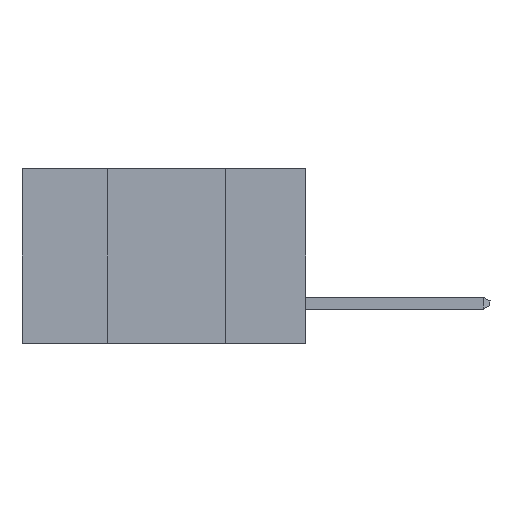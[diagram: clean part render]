
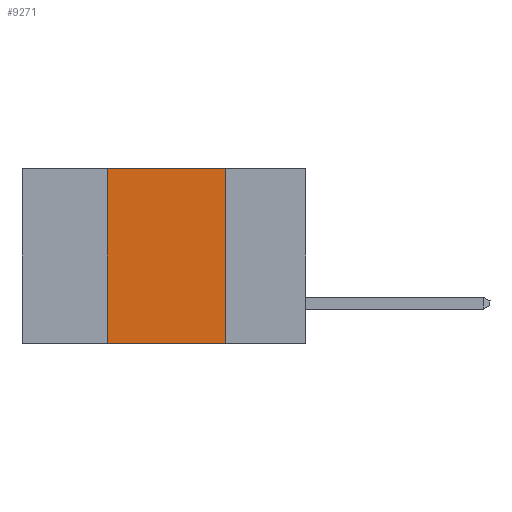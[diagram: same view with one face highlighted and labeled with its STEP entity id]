
A CAD part, left-side view. The second image highlights one B-rep face of the part: STEP entity #9271.
In plain terms, the highlighted planar face has unit normal (-1, 0, 0).
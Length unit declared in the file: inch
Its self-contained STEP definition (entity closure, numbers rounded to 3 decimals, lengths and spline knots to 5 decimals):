
#103 = DIRECTION ( 'NONE',  ( 0., 0., -1. ) ) ;
#150 = DIRECTION ( 'NONE',  ( 0., -1., 0. ) ) ;
#769 = CARTESIAN_POINT ( 'NONE',  ( 0., 0.17, -0.37 ) ) ;
#1014 = LINE ( 'NONE', #6149, #9701 ) ;
#1669 = VERTEX_POINT ( 'NONE', #7703 ) ;
#1776 = ORIENTED_EDGE ( 'NONE', *, *, #10661, .F. ) ;
#2190 = DIRECTION ( 'NONE',  ( 0., 0., 1. ) ) ;
#2389 = ORIENTED_EDGE ( 'NONE', *, *, #3791, .T. ) ;
#2698 = VECTOR ( 'NONE', #2190, 39.37008 ) ;
#3248 = FACE_OUTER_BOUND ( 'NONE', #10549, .T. ) ;
#3507 = CARTESIAN_POINT ( 'NONE',  ( 0., 0.42, -0.37 ) ) ;
#3791 = EDGE_CURVE ( 'NONE', #6708, #4598, #1014, .T. ) ;
#3849 = LINE ( 'NONE', #7345, #8495 ) ;
#4230 = DIRECTION ( 'NONE',  ( 0., 0., -1. ) ) ;
#4333 = VERTEX_POINT ( 'NONE', #9181 ) ;
#4598 = VERTEX_POINT ( 'NONE', #769 ) ;
#4929 = EDGE_CURVE ( 'NONE', #6708, #4333, #8360, .T. ) ;
#5251 = ORIENTED_EDGE ( 'NONE', *, *, #4929, .F. ) ;
#5460 = CARTESIAN_POINT ( 'NONE',  ( 0., 0.17, -0.37 ) ) ;
#6149 = CARTESIAN_POINT ( 'NONE',  ( 0., 0.6, -0.37 ) ) ;
#6198 = ORIENTED_EDGE ( 'NONE', *, *, #8192, .F. ) ;
#6570 = CARTESIAN_POINT ( 'NONE',  ( 0., 0.42, -0.37 ) ) ;
#6708 = VERTEX_POINT ( 'NONE', #3507 ) ;
#7345 = CARTESIAN_POINT ( 'NONE',  ( 0., 0.6, 0. ) ) ;
#7703 = CARTESIAN_POINT ( 'NONE',  ( 0., 0.17, 0. ) ) ;
#7717 = AXIS2_PLACEMENT_3D ( 'NONE', #7826, #11349, #4230 ) ;
#7826 = CARTESIAN_POINT ( 'NONE',  ( 0., 0.6, 0. ) ) ;
#8192 = EDGE_CURVE ( 'NONE', #1669, #4598, #9153, .T. ) ;
#8360 = LINE ( 'NONE', #6570, #2698 ) ;
#8495 = VECTOR ( 'NONE', #10861, 39.37008 ) ;
#8551 = PLANE ( 'NONE',  #7717 ) ;
#9153 = LINE ( 'NONE', #5460, #11037 ) ;
#9181 = CARTESIAN_POINT ( 'NONE',  ( 0., 0.42, 0. ) ) ;
#9271 = ADVANCED_FACE ( 'NONE', ( #3248 ), #8551, .F. ) ;
#9701 = VECTOR ( 'NONE', #150, 39.37008 ) ;
#10549 = EDGE_LOOP ( 'NONE', ( #6198, #1776, #5251, #2389 ) ) ;
#10661 = EDGE_CURVE ( 'NONE', #4333, #1669, #3849, .T. ) ;
#10861 = DIRECTION ( 'NONE',  ( 0., -1., 0. ) ) ;
#11037 = VECTOR ( 'NONE', #103, 39.37008 ) ;
#11349 = DIRECTION ( 'NONE',  ( 1., 0., 0. ) ) ;
